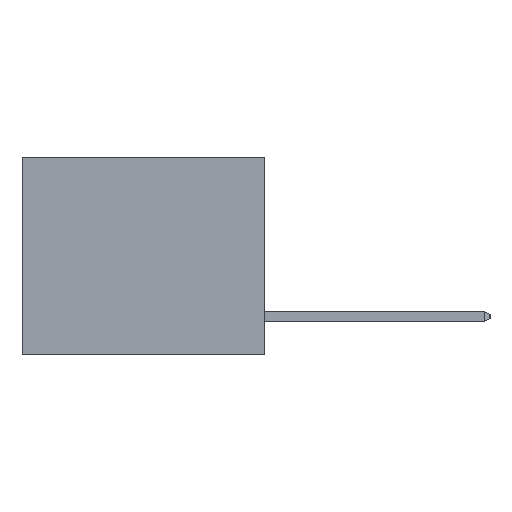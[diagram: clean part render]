
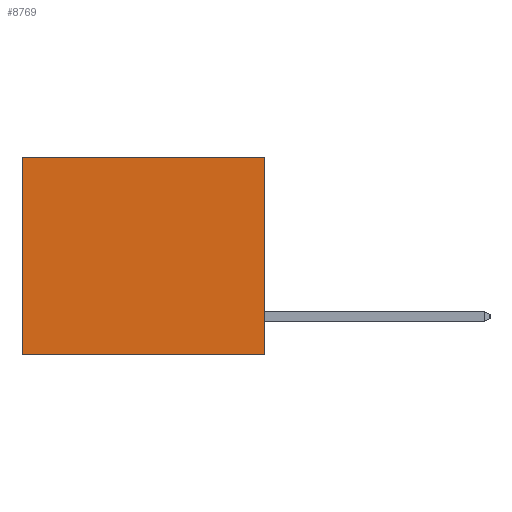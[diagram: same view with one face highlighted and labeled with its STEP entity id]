
A CAD part, left-side view. The second image highlights one B-rep face of the part: STEP entity #8769.
In plain terms, the highlighted planar face has unit normal (-1, 0, 0).
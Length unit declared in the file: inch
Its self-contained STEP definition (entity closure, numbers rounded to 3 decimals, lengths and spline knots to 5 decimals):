
#365 = CARTESIAN_POINT ( 'NONE',  ( 0.3165, 0.6, -0.49 ) ) ;
#1426 = VERTEX_POINT ( 'NONE', #10244 ) ;
#1539 = EDGE_CURVE ( 'NONE', #7231, #1426, #2495, .T. ) ;
#1570 = FACE_OUTER_BOUND ( 'NONE', #4889, .T. ) ;
#1947 = PLANE ( 'NONE',  #9758 ) ;
#2100 = EDGE_CURVE ( 'NONE', #4346, #6472, #7629, .T. ) ;
#2495 = LINE ( 'NONE', #9453, #2867 ) ;
#2613 = ORIENTED_EDGE ( 'NONE', *, *, #1539, .F. ) ;
#2807 = DIRECTION ( 'NONE',  ( 0., 0., -1. ) ) ;
#2867 = VECTOR ( 'NONE', #6111, 39.37008 ) ;
#3461 = CARTESIAN_POINT ( 'NONE',  ( 0.3165, 0., -0.49 ) ) ;
#3541 = LINE ( 'NONE', #9115, #5457 ) ;
#3811 = EDGE_CURVE ( 'NONE', #7231, #4346, #7521, .T. ) ;
#4346 = VERTEX_POINT ( 'NONE', #9633 ) ;
#4889 = EDGE_LOOP ( 'NONE', ( #6816, #6262, #2613, #4932 ) ) ;
#4932 = ORIENTED_EDGE ( 'NONE', *, *, #3811, .T. ) ;
#5272 = CARTESIAN_POINT ( 'NONE',  ( 0.3165, 0.6, -0.49 ) ) ;
#5457 = VECTOR ( 'NONE', #9194, 39.37008 ) ;
#5771 = CARTESIAN_POINT ( 'NONE',  ( 0.3165, 0., 0. ) ) ;
#6026 = DIRECTION ( 'NONE',  ( 1., 0., 0. ) ) ;
#6111 = DIRECTION ( 'NONE',  ( 0., 0., -1. ) ) ;
#6262 = ORIENTED_EDGE ( 'NONE', *, *, #9887, .F. ) ;
#6472 = VERTEX_POINT ( 'NONE', #365 ) ;
#6816 = ORIENTED_EDGE ( 'NONE', *, *, #2100, .T. ) ;
#7231 = VERTEX_POINT ( 'NONE', #8981 ) ;
#7521 = LINE ( 'NONE', #5771, #10441 ) ;
#7597 = DIRECTION ( 'NONE',  ( 0., 0., -1. ) ) ;
#7629 = LINE ( 'NONE', #5272, #9300 ) ;
#8040 = DIRECTION ( 'NONE',  ( 0., 1., 0. ) ) ;
#8769 = ADVANCED_FACE ( 'NONE', ( #1570 ), #1947, .F. ) ;
#8981 = CARTESIAN_POINT ( 'NONE',  ( 0.3165, 0., 0. ) ) ;
#9115 = CARTESIAN_POINT ( 'NONE',  ( 0.3165, 0., -0.49 ) ) ;
#9194 = DIRECTION ( 'NONE',  ( 0., 1., 0. ) ) ;
#9300 = VECTOR ( 'NONE', #7597, 39.37008 ) ;
#9453 = CARTESIAN_POINT ( 'NONE',  ( 0.3165, 0., -0.49 ) ) ;
#9633 = CARTESIAN_POINT ( 'NONE',  ( 0.3165, 0.6, 0. ) ) ;
#9758 = AXIS2_PLACEMENT_3D ( 'NONE', #3461, #6026, #2807 ) ;
#9887 = EDGE_CURVE ( 'NONE', #1426, #6472, #3541, .T. ) ;
#10244 = CARTESIAN_POINT ( 'NONE',  ( 0.3165, 0., -0.49 ) ) ;
#10441 = VECTOR ( 'NONE', #8040, 39.37008 ) ;
